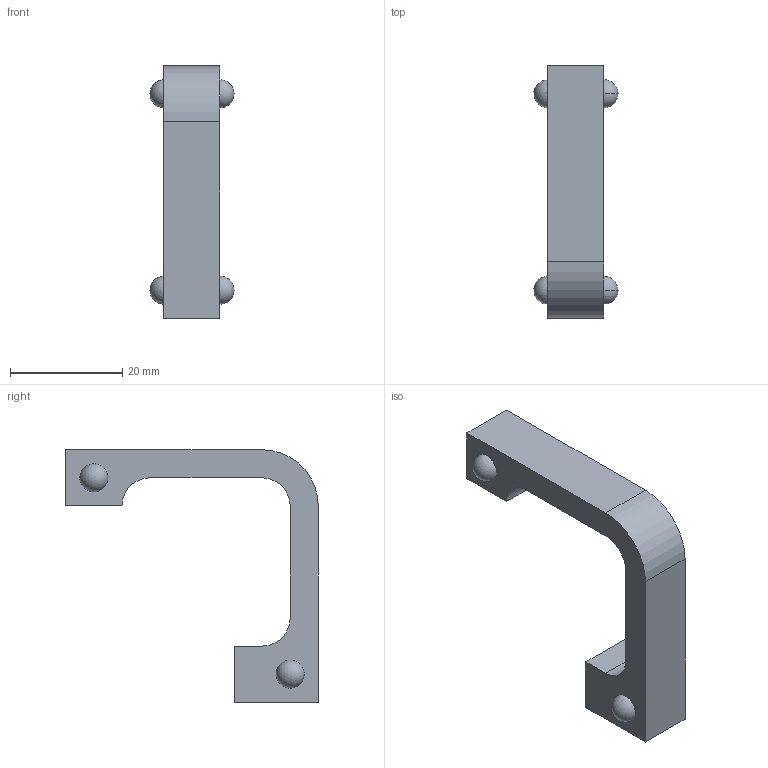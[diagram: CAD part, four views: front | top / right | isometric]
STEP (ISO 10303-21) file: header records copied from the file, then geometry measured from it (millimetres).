
FILE_DESCRIPTION (( 'STEP AP214' ), '1' );
FILE_NAME ('Trigger_Guard_Front.step', '2013-11-06T14:31:44', ( 'elpi' ), ( '' ), 'SwSTEP 2.0', 'SolidWorks 2013', '' );
FILE_SCHEMA (( 'AUTOMOTIVE_DESIGN' ));
Length unit declared in the file: millimetre
Products named in the file (1): Trigger_Guard_Front
Bounding box: 14.98 x 45 x 45 mm (x, y, z)
Volume: 5827.2 mm3; surface area: 3210.5 mm2
Topology: 1 solids, 1 shells, 21 faces, 65 edges, 42 vertices
Faces by surface type: plane 11, sphere 6, cylinder 4
Entity records: 647 total; most frequent: DIRECTION 111, CARTESIAN_POINT 105, ORIENTED_EDGE 98, EDGE_CURVE 49, AXIS2_PLACEMENT_3D 40, VERTEX_POINT 34, VECTOR 31, LINE 31
